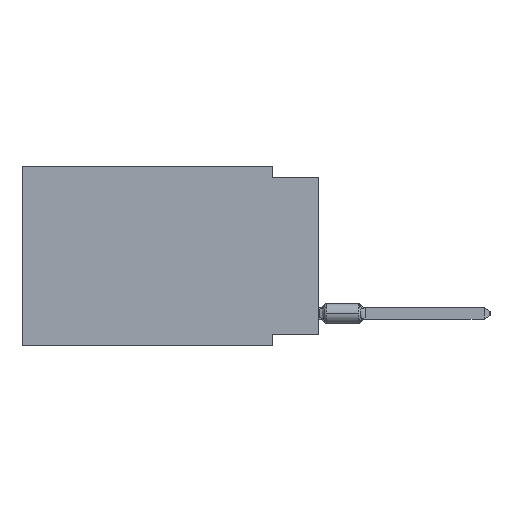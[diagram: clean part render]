
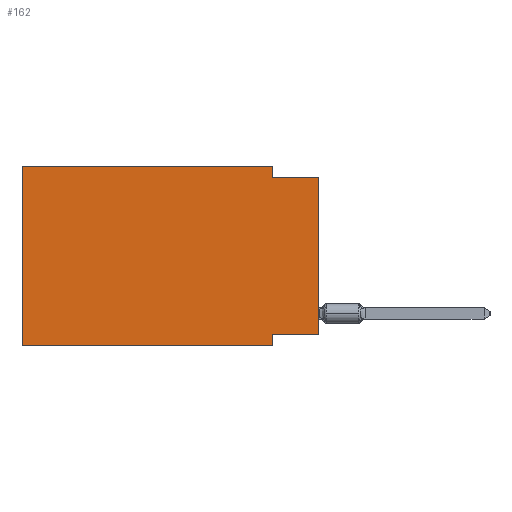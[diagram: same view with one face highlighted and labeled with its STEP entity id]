
A CAD part, left-side view. The second image highlights one B-rep face of the part: STEP entity #162.
In plain terms, the highlighted planar face has unit normal (-1, 0, 0).
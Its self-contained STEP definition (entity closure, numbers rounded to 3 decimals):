
#72 = VERTEX_POINT ( 'NONE', #45521 ) ;
#162 = ADVANCED_FACE ( 'NONE', ( #51808 ), #18183, .F. ) ;
#436 = DIRECTION ( 'NONE',  ( 0., 0., -1. ) ) ;
#1720 = CARTESIAN_POINT ( 'NONE',  ( 0., 16.383, 0. ) ) ;
#2789 = VECTOR ( 'NONE', #40338, 1000. ) ;
#4530 = VECTOR ( 'NONE', #24951, 1000. ) ;
#5935 = DIRECTION ( 'NONE',  ( 0., 1., 0. ) ) ;
#6105 = LINE ( 'NONE', #12002, #34987 ) ;
#7593 = EDGE_CURVE ( 'NONE', #21015, #72, #69174, .T. ) ;
#7853 = CARTESIAN_POINT ( 'NONE',  ( 0., 0., -9.271 ) ) ;
#8695 = CARTESIAN_POINT ( 'NONE',  ( 0., 2.54, -9.906 ) ) ;
#10102 = AXIS2_PLACEMENT_3D ( 'NONE', #24462, #35535, #29623 ) ;
#10248 = VECTOR ( 'NONE', #40367, 1000. ) ;
#10719 = VECTOR ( 'NONE', #65974, 1000. ) ;
#12002 = CARTESIAN_POINT ( 'NONE',  ( 0., 16.383, 0. ) ) ;
#12433 = VECTOR ( 'NONE', #436, 1000. ) ;
#12643 = CARTESIAN_POINT ( 'NONE',  ( 0., 16.383, -9.906 ) ) ;
#12699 = VECTOR ( 'NONE', #5935, 1000. ) ;
#12763 = DIRECTION ( 'NONE',  ( 0., 0., 1. ) ) ;
#18183 = PLANE ( 'NONE',  #10102 ) ;
#18184 = LINE ( 'NONE', #12643, #65624 ) ;
#21015 = VERTEX_POINT ( 'NONE', #30585 ) ;
#21347 = EDGE_CURVE ( 'NONE', #35460, #45463, #18184, .T. ) ;
#22887 = EDGE_CURVE ( 'NONE', #44283, #56845, #49912, .T. ) ;
#22966 = LINE ( 'NONE', #43426, #10719 ) ;
#23279 = CARTESIAN_POINT ( 'NONE',  ( 0., 0., -9.271 ) ) ;
#24462 = CARTESIAN_POINT ( 'NONE',  ( 0., 16.383, 0. ) ) ;
#24536 = VERTEX_POINT ( 'NONE', #57190 ) ;
#24951 = DIRECTION ( 'NONE',  ( 0., -1., 0. ) ) ;
#29623 = DIRECTION ( 'NONE',  ( 0., 0., -1. ) ) ;
#30585 = CARTESIAN_POINT ( 'NONE',  ( 0., 2.54, 0. ) ) ;
#32957 = EDGE_CURVE ( 'NONE', #35460, #35309, #6105, .T. ) ;
#33434 = EDGE_CURVE ( 'NONE', #44283, #24536, #50734, .T. ) ;
#33662 = LINE ( 'NONE', #56218, #12433 ) ;
#34453 = CARTESIAN_POINT ( 'NONE',  ( 0., 0., 0. ) ) ;
#34987 = VECTOR ( 'NONE', #12763, 1000. ) ;
#35309 = VERTEX_POINT ( 'NONE', #59829 ) ;
#35460 = VERTEX_POINT ( 'NONE', #63114 ) ;
#35535 = DIRECTION ( 'NONE',  ( 1., 0., 0. ) ) ;
#36040 = LINE ( 'NONE', #1720, #4530 ) ;
#40338 = DIRECTION ( 'NONE',  ( 0., 0., -1. ) ) ;
#40367 = DIRECTION ( 'NONE',  ( 0., 0., 1. ) ) ;
#41567 = ORIENTED_EDGE ( 'NONE', *, *, #33434, .T. ) ;
#43426 = CARTESIAN_POINT ( 'NONE',  ( 0., 0., -0.635 ) ) ;
#44283 = VERTEX_POINT ( 'NONE', #7853 ) ;
#45325 = CARTESIAN_POINT ( 'NONE',  ( 0., 2.54, -9.271 ) ) ;
#45463 = VERTEX_POINT ( 'NONE', #8695 ) ;
#45521 = CARTESIAN_POINT ( 'NONE',  ( 0., 2.54, -0.635 ) ) ;
#47558 = ORIENTED_EDGE ( 'NONE', *, *, #64270, .F. ) ;
#49264 = EDGE_CURVE ( 'NONE', #56845, #45463, #33662, .T. ) ;
#49912 = LINE ( 'NONE', #23279, #12699 ) ;
#50734 = LINE ( 'NONE', #34453, #10248 ) ;
#51423 = EDGE_LOOP ( 'NONE', ( #41567, #64310, #61087, #47558, #54012, #51796, #57236, #68288 ) ) ;
#51796 = ORIENTED_EDGE ( 'NONE', *, *, #21347, .T. ) ;
#51808 = FACE_OUTER_BOUND ( 'NONE', #51423, .T. ) ;
#54012 = ORIENTED_EDGE ( 'NONE', *, *, #32957, .F. ) ;
#56218 = CARTESIAN_POINT ( 'NONE',  ( 0., 2.54, -9.906 ) ) ;
#56621 = DIRECTION ( 'NONE',  ( 0., -1., 0. ) ) ;
#56845 = VERTEX_POINT ( 'NONE', #45325 ) ;
#57190 = CARTESIAN_POINT ( 'NONE',  ( 0., 0., -0.635 ) ) ;
#57236 = ORIENTED_EDGE ( 'NONE', *, *, #49264, .F. ) ;
#59829 = CARTESIAN_POINT ( 'NONE',  ( 0., 16.383, 0. ) ) ;
#61087 = ORIENTED_EDGE ( 'NONE', *, *, #7593, .F. ) ;
#62523 = CARTESIAN_POINT ( 'NONE',  ( 0., 2.54, 0. ) ) ;
#63114 = CARTESIAN_POINT ( 'NONE',  ( 0., 16.383, -9.906 ) ) ;
#64270 = EDGE_CURVE ( 'NONE', #35309, #21015, #36040, .T. ) ;
#64310 = ORIENTED_EDGE ( 'NONE', *, *, #67263, .F. ) ;
#65624 = VECTOR ( 'NONE', #56621, 1000. ) ;
#65974 = DIRECTION ( 'NONE',  ( 0., -1., 0. ) ) ;
#67263 = EDGE_CURVE ( 'NONE', #72, #24536, #22966, .T. ) ;
#68288 = ORIENTED_EDGE ( 'NONE', *, *, #22887, .F. ) ;
#69174 = LINE ( 'NONE', #62523, #2789 ) ;
